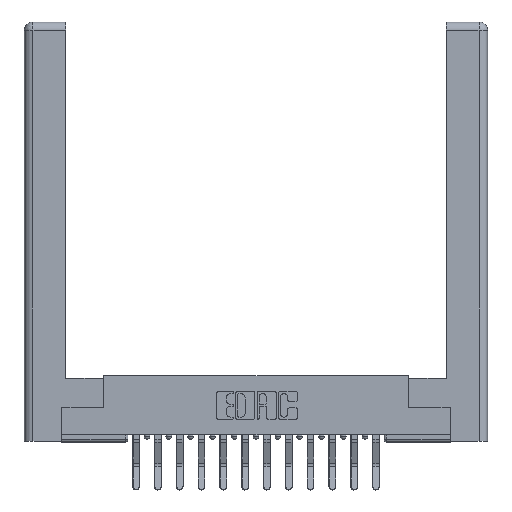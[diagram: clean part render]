
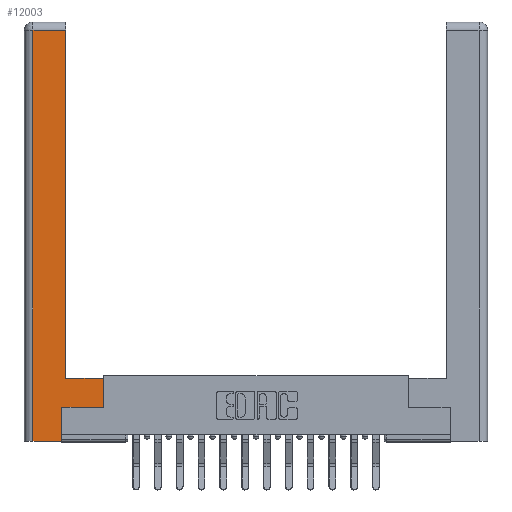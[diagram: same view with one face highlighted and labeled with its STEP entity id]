
A CAD part, top view. The second image highlights one B-rep face of the part: STEP entity #12003.
In plain terms, the highlighted planar face has unit normal (0, 0, 1).
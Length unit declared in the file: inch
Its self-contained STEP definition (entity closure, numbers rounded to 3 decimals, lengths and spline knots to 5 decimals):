
#161 = VECTOR ( 'NONE', #13018, 39.37008 ) ;
#188 = VERTEX_POINT ( 'NONE', #9186 ) ;
#613 = CARTESIAN_POINT ( 'NONE',  ( 0.295, 3., 0. ) ) ;
#896 = CARTESIAN_POINT ( 'NONE',  ( 0.565, 0.245, 0. ) ) ;
#1011 = DIRECTION ( 'NONE',  ( 0., -1., 0. ) ) ;
#1836 = EDGE_CURVE ( 'NONE', #6236, #6061, #10845, .T. ) ;
#2224 = DIRECTION ( 'NONE',  ( -1., 0., 0. ) ) ;
#2371 = ORIENTED_EDGE ( 'NONE', *, *, #1836, .T. ) ;
#2516 = CARTESIAN_POINT ( 'NONE',  ( 0.565, 0.45, 0. ) ) ;
#3198 = LINE ( 'NONE', #613, #13748 ) ;
#3651 = CARTESIAN_POINT ( 'NONE',  ( 0.0615, 2.94, 0. ) ) ;
#3708 = AXIS2_PLACEMENT_3D ( 'NONE', #10749, #12128, #5631 ) ;
#3829 = EDGE_CURVE ( 'NONE', #11496, #12694, #9554, .T. ) ;
#3978 = VERTEX_POINT ( 'NONE', #14446 ) ;
#4032 = LINE ( 'NONE', #896, #11082 ) ;
#4384 = DIRECTION ( 'NONE',  ( 1., 0., 0. ) ) ;
#4439 = CARTESIAN_POINT ( 'NONE',  ( 0.265, 0., 0. ) ) ;
#4451 = ORIENTED_EDGE ( 'NONE', *, *, #16588, .T. ) ;
#5109 = EDGE_LOOP ( 'NONE', ( #11379, #5750, #16237, #12853, #2371, #4451, #9860, #5546 ) ) ;
#5297 = VECTOR ( 'NONE', #4384, 39.37008 ) ;
#5408 = FACE_OUTER_BOUND ( 'NONE', #5109, .T. ) ;
#5546 = ORIENTED_EDGE ( 'NONE', *, *, #7251, .T. ) ;
#5631 = DIRECTION ( 'NONE',  ( -1., 0., 0. ) ) ;
#5750 = ORIENTED_EDGE ( 'NONE', *, *, #3829, .T. ) ;
#5804 = EDGE_CURVE ( 'NONE', #12799, #188, #15283, .T. ) ;
#6061 = VERTEX_POINT ( 'NONE', #8287 ) ;
#6236 = VERTEX_POINT ( 'NONE', #4439 ) ;
#6980 = LINE ( 'NONE', #7607, #12578 ) ;
#7238 = DIRECTION ( 'NONE',  ( 0., 1., 0. ) ) ;
#7251 = EDGE_CURVE ( 'NONE', #188, #16642, #7551, .T. ) ;
#7486 = DIRECTION ( 'NONE',  ( 1., 0., 0. ) ) ;
#7551 = LINE ( 'NONE', #16167, #10673 ) ;
#7607 = CARTESIAN_POINT ( 'NONE',  ( 0.0615, 0., 0. ) ) ;
#8115 = CARTESIAN_POINT ( 'NONE',  ( 0.0615, 2.94, 0. ) ) ;
#8287 = CARTESIAN_POINT ( 'NONE',  ( 0.265, 0.245, 0. ) ) ;
#8315 = EDGE_CURVE ( 'NONE', #12694, #3978, #6980, .T. ) ;
#8449 = CARTESIAN_POINT ( 'NONE',  ( 0.265, 0., 0. ) ) ;
#9186 = CARTESIAN_POINT ( 'NONE',  ( 0.565, 0.45, 0. ) ) ;
#9193 = PLANE ( 'NONE',  #3708 ) ;
#9554 = LINE ( 'NONE', #3651, #11835 ) ;
#9572 = CARTESIAN_POINT ( 'NONE',  ( 0.565, 0.245, 0. ) ) ;
#9860 = ORIENTED_EDGE ( 'NONE', *, *, #5804, .T. ) ;
#10673 = VECTOR ( 'NONE', #12058, 39.37008 ) ;
#10691 = EDGE_CURVE ( 'NONE', #16642, #11496, #3198, .T. ) ;
#10749 = CARTESIAN_POINT ( 'NONE',  ( 0., 0., 0. ) ) ;
#10845 = LINE ( 'NONE', #17110, #12888 ) ;
#11082 = VECTOR ( 'NONE', #7486, 39.37008 ) ;
#11379 = ORIENTED_EDGE ( 'NONE', *, *, #10691, .T. ) ;
#11496 = VERTEX_POINT ( 'NONE', #13642 ) ;
#11835 = VECTOR ( 'NONE', #2224, 39.37008 ) ;
#12003 = ADVANCED_FACE ( 'NONE', ( #5408 ), #9193, .F. ) ;
#12058 = DIRECTION ( 'NONE',  ( -1., 0., 0. ) ) ;
#12128 = DIRECTION ( 'NONE',  ( 0., 0., -1. ) ) ;
#12578 = VECTOR ( 'NONE', #1011, 39.37008 ) ;
#12694 = VERTEX_POINT ( 'NONE', #8115 ) ;
#12799 = VERTEX_POINT ( 'NONE', #9572 ) ;
#12853 = ORIENTED_EDGE ( 'NONE', *, *, #15953, .T. ) ;
#12888 = VECTOR ( 'NONE', #14509, 39.37008 ) ;
#13018 = DIRECTION ( 'NONE',  ( 0., 1., 0. ) ) ;
#13380 = LINE ( 'NONE', #8449, #5297 ) ;
#13642 = CARTESIAN_POINT ( 'NONE',  ( 0.295, 2.94, 0. ) ) ;
#13748 = VECTOR ( 'NONE', #7238, 39.37008 ) ;
#14446 = CARTESIAN_POINT ( 'NONE',  ( 0.0615, 0., 0. ) ) ;
#14509 = DIRECTION ( 'NONE',  ( 0., 1., 0. ) ) ;
#15283 = LINE ( 'NONE', #2516, #161 ) ;
#15953 = EDGE_CURVE ( 'NONE', #3978, #6236, #13380, .T. ) ;
#16167 = CARTESIAN_POINT ( 'NONE',  ( 0.295, 0.45, 0. ) ) ;
#16237 = ORIENTED_EDGE ( 'NONE', *, *, #8315, .T. ) ;
#16588 = EDGE_CURVE ( 'NONE', #6061, #12799, #4032, .T. ) ;
#16642 = VERTEX_POINT ( 'NONE', #16687 ) ;
#16687 = CARTESIAN_POINT ( 'NONE',  ( 0.295, 0.45, 0. ) ) ;
#17110 = CARTESIAN_POINT ( 'NONE',  ( 0.265, 0.245, 0. ) ) ;
